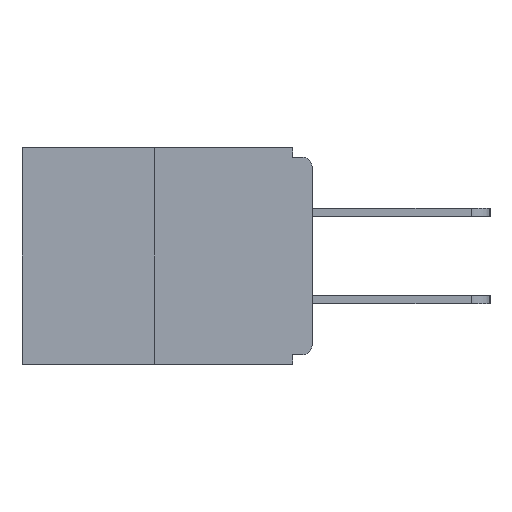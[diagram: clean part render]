
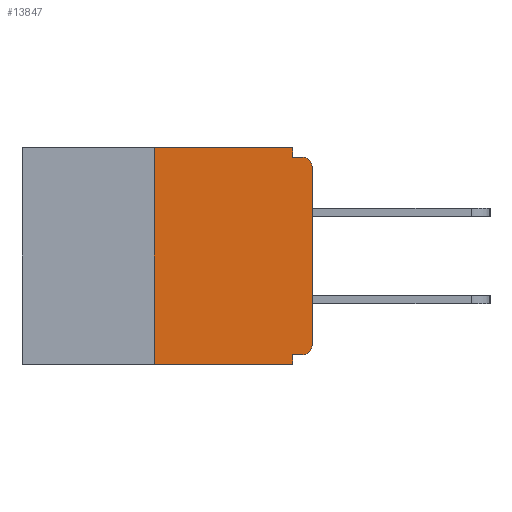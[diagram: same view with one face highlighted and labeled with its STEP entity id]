
A CAD part, left-side view. The second image highlights one B-rep face of the part: STEP entity #13847.
In plain terms, the highlighted planar face has unit normal (-1, 0, 0).
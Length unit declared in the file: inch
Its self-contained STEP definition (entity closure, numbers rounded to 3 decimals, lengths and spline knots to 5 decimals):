
#74 = LINE ( 'NONE', #15976, #10434 ) ;
#445 = ORIENTED_EDGE ( 'NONE', *, *, #2252, .F. ) ;
#1049 = VERTEX_POINT ( 'NONE', #4028 ) ;
#1458 = AXIS2_PLACEMENT_3D ( 'NONE', #8008, #1974, #11416 ) ;
#1469 = EDGE_LOOP ( 'NONE', ( #14645, #8441, #8454, #15903, #7942, #14533, #8207, #11943, #445, #6150 ) ) ;
#1935 = VERTEX_POINT ( 'NONE', #2079 ) ;
#1974 = DIRECTION ( 'NONE',  ( -1., 0., 0. ) ) ;
#2079 = CARTESIAN_POINT ( 'NONE',  ( 0., 0.031, -0.343 ) ) ;
#2250 = PLANE ( 'NONE',  #4190 ) ;
#2252 = EDGE_CURVE ( 'NONE', #15812, #2888, #11798, .T. ) ;
#2888 = VERTEX_POINT ( 'NONE', #20257 ) ;
#3229 = DIRECTION ( 'NONE',  ( 0., -1., 0. ) ) ;
#3465 = EDGE_CURVE ( 'NONE', #8174, #18782, #14973, .T. ) ;
#3678 = CARTESIAN_POINT ( 'NONE',  ( 0., 0.031, -0.015 ) ) ;
#4028 = CARTESIAN_POINT ( 'NONE',  ( 0., 0.25, 0. ) ) ;
#4190 = AXIS2_PLACEMENT_3D ( 'NONE', #19981, #10007, #15081 ) ;
#4297 = DIRECTION ( 'NONE',  ( -1., 0., 0. ) ) ;
#4587 = CARTESIAN_POINT ( 'NONE',  ( 0., 0.25, -0.343 ) ) ;
#4757 = VECTOR ( 'NONE', #7690, 39.37008 ) ;
#4928 = DIRECTION ( 'NONE',  ( 0., 0., 1. ) ) ;
#5178 = CIRCLE ( 'NONE', #1458, 0.015 ) ;
#5703 = EDGE_CURVE ( 'NONE', #8174, #12635, #12729, .T. ) ;
#5875 = EDGE_CURVE ( 'NONE', #11705, #1049, #5980, .T. ) ;
#5970 = VECTOR ( 'NONE', #3229, 39.37008 ) ;
#5980 = LINE ( 'NONE', #16586, #14173 ) ;
#6150 = ORIENTED_EDGE ( 'NONE', *, *, #11172, .F. ) ;
#6272 = AXIS2_PLACEMENT_3D ( 'NONE', #12360, #4297, #10796 ) ;
#6401 = CARTESIAN_POINT ( 'NONE',  ( 0., 0., 0. ) ) ;
#6613 = CARTESIAN_POINT ( 'NONE',  ( 0., 0.46, 0. ) ) ;
#7690 = DIRECTION ( 'NONE',  ( 0., 0., -1. ) ) ;
#7942 = ORIENTED_EDGE ( 'NONE', *, *, #3465, .F. ) ;
#8008 = CARTESIAN_POINT ( 'NONE',  ( 0., 0.015, -0.03 ) ) ;
#8174 = VERTEX_POINT ( 'NONE', #19518 ) ;
#8207 = ORIENTED_EDGE ( 'NONE', *, *, #19964, .T. ) ;
#8441 = ORIENTED_EDGE ( 'NONE', *, *, #5875, .F. ) ;
#8454 = ORIENTED_EDGE ( 'NONE', *, *, #11794, .T. ) ;
#8586 = CARTESIAN_POINT ( 'NONE',  ( 0., 0., -0.015 ) ) ;
#8831 = VERTEX_POINT ( 'NONE', #19909 ) ;
#9308 = DIRECTION ( 'NONE',  ( 0., 0., -1. ) ) ;
#9691 = LINE ( 'NONE', #16151, #15618 ) ;
#9805 = LINE ( 'NONE', #6613, #5970 ) ;
#9991 = VECTOR ( 'NONE', #18587, 39.37008 ) ;
#10007 = DIRECTION ( 'NONE',  ( 1., 0., 0. ) ) ;
#10106 = DIRECTION ( 'NONE',  ( 0., -1., 0. ) ) ;
#10434 = VECTOR ( 'NONE', #9308, 39.37008 ) ;
#10796 = DIRECTION ( 'NONE',  ( 0., 0., -1. ) ) ;
#11003 = LINE ( 'NONE', #19165, #4757 ) ;
#11172 = EDGE_CURVE ( 'NONE', #12201, #15812, #11003, .T. ) ;
#11398 = DIRECTION ( 'NONE',  ( 0., 0., 1. ) ) ;
#11416 = DIRECTION ( 'NONE',  ( 0., 0., -1. ) ) ;
#11491 = DIRECTION ( 'NONE',  ( 0., -1., 0. ) ) ;
#11705 = VERTEX_POINT ( 'NONE', #4587 ) ;
#11794 = EDGE_CURVE ( 'NONE', #11705, #1935, #9691, .T. ) ;
#11798 = LINE ( 'NONE', #8586, #19715 ) ;
#11943 = ORIENTED_EDGE ( 'NONE', *, *, #13267, .T. ) ;
#12201 = VERTEX_POINT ( 'NONE', #20776 ) ;
#12360 = CARTESIAN_POINT ( 'NONE',  ( 0., 0.015, -0.313 ) ) ;
#12635 = VERTEX_POINT ( 'NONE', #18053 ) ;
#12729 = CIRCLE ( 'NONE', #6272, 0.015 ) ;
#13267 = EDGE_CURVE ( 'NONE', #8831, #2888, #5178, .T. ) ;
#13847 = ADVANCED_FACE ( 'NONE', ( #20078 ), #2250, .F. ) ;
#14149 = LINE ( 'NONE', #6401, #17719 ) ;
#14173 = VECTOR ( 'NONE', #4928, 39.37008 ) ;
#14533 = ORIENTED_EDGE ( 'NONE', *, *, #5703, .T. ) ;
#14645 = ORIENTED_EDGE ( 'NONE', *, *, #16787, .F. ) ;
#14973 = LINE ( 'NONE', #18267, #9991 ) ;
#15081 = DIRECTION ( 'NONE',  ( 0., 0., -1. ) ) ;
#15618 = VECTOR ( 'NONE', #11491, 39.37008 ) ;
#15812 = VERTEX_POINT ( 'NONE', #3678 ) ;
#15903 = ORIENTED_EDGE ( 'NONE', *, *, #18250, .F. ) ;
#15976 = CARTESIAN_POINT ( 'NONE',  ( 0., 0.031, -0.343 ) ) ;
#16151 = CARTESIAN_POINT ( 'NONE',  ( 0., 0.46, -0.343 ) ) ;
#16369 = CARTESIAN_POINT ( 'NONE',  ( 0., 0.031, -0.328 ) ) ;
#16586 = CARTESIAN_POINT ( 'NONE',  ( 0., 0.25, 0. ) ) ;
#16787 = EDGE_CURVE ( 'NONE', #1049, #12201, #9805, .T. ) ;
#17719 = VECTOR ( 'NONE', #11398, 39.37008 ) ;
#18053 = CARTESIAN_POINT ( 'NONE',  ( 0., 0., -0.313 ) ) ;
#18250 = EDGE_CURVE ( 'NONE', #18782, #1935, #74, .T. ) ;
#18267 = CARTESIAN_POINT ( 'NONE',  ( 0., 0., -0.328 ) ) ;
#18587 = DIRECTION ( 'NONE',  ( 0., 1., 0. ) ) ;
#18782 = VERTEX_POINT ( 'NONE', #16369 ) ;
#19165 = CARTESIAN_POINT ( 'NONE',  ( 0., 0.031, 0. ) ) ;
#19518 = CARTESIAN_POINT ( 'NONE',  ( 0., 0.015, -0.328 ) ) ;
#19715 = VECTOR ( 'NONE', #10106, 39.37008 ) ;
#19909 = CARTESIAN_POINT ( 'NONE',  ( 0., 0., -0.03 ) ) ;
#19964 = EDGE_CURVE ( 'NONE', #12635, #8831, #14149, .T. ) ;
#19981 = CARTESIAN_POINT ( 'NONE',  ( 0., 0.46, 0. ) ) ;
#20078 = FACE_OUTER_BOUND ( 'NONE', #1469, .T. ) ;
#20257 = CARTESIAN_POINT ( 'NONE',  ( 0., 0.015, -0.015 ) ) ;
#20776 = CARTESIAN_POINT ( 'NONE',  ( 0., 0.031, 0. ) ) ;
